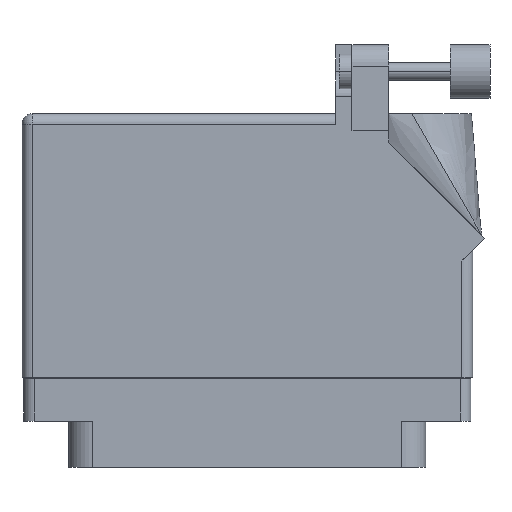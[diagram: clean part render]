
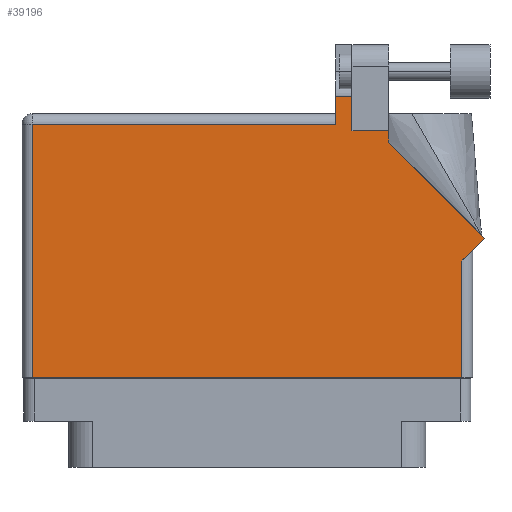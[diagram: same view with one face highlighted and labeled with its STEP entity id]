
A CAD part, front view. The second image highlights one B-rep face of the part: STEP entity #39196.
In plain terms, the highlighted face is planar.
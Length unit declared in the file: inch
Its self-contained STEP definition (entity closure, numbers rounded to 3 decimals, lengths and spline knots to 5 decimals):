
#301 = EDGE_CURVE ( 'NONE', #4619, #9848, #6210, .T. ) ;
#401 = DIRECTION ( 'NONE',  ( -1., 0., 0. ) ) ;
#438 = ORIENTED_EDGE ( 'NONE', *, *, #20001, .T. ) ;
#2689 = DIRECTION ( 'NONE',  ( 0., 1., 0. ) ) ;
#3340 = FACE_OUTER_BOUND ( 'NONE', #44465, .T. ) ;
#3405 = VECTOR ( 'NONE', #4112, 39.37008 ) ;
#3554 = EDGE_CURVE ( 'NONE', #15527, #26384, #39016, .T. ) ;
#4112 = DIRECTION ( 'NONE',  ( -1., 0., 0. ) ) ;
#4385 = ORIENTED_EDGE ( 'NONE', *, *, #27018, .T. ) ;
#4619 = VERTEX_POINT ( 'NONE', #20329 ) ;
#5492 = DIRECTION ( 'NONE',  ( 0.707, 0.707, 0. ) ) ;
#5613 = DIRECTION ( 'NONE',  ( -1., 0., 0. ) ) ;
#6042 = DIRECTION ( 'NONE',  ( -0.707, 0.707, 0. ) ) ;
#6210 = LINE ( 'NONE', #43360, #33582 ) ;
#6911 = EDGE_CURVE ( 'NONE', #28225, #24283, #7687, .T. ) ;
#7637 = VECTOR ( 'NONE', #14661, 39.37008 ) ;
#7687 = LINE ( 'NONE', #38793, #29189 ) ;
#8097 = LINE ( 'NONE', #26347, #3405 ) ;
#8151 = LINE ( 'NONE', #30465, #29691 ) ;
#9648 = ORIENTED_EDGE ( 'NONE', *, *, #18750, .T. ) ;
#9848 = VERTEX_POINT ( 'NONE', #14142 ) ;
#10163 = VECTOR ( 'NONE', #5492, 39.37008 ) ;
#10864 = ORIENTED_EDGE ( 'NONE', *, *, #29958, .T. ) ;
#11469 = LINE ( 'NONE', #13378, #44058 ) ;
#11847 = AXIS2_PLACEMENT_3D ( 'NONE', #15701, #12307, #5613 ) ;
#12105 = EDGE_CURVE ( 'NONE', #9848, #18011, #33276, .T. ) ;
#12145 = ORIENTED_EDGE ( 'NONE', *, *, #34560, .T. ) ;
#12307 = DIRECTION ( 'NONE',  ( 0., 0., -1. ) ) ;
#13378 = CARTESIAN_POINT ( 'NONE',  ( 1.37671, 0.70771, 0.455 ) ) ;
#13670 = CARTESIAN_POINT ( 'NONE',  ( 1.244, 0.575, 0.455 ) ) ;
#13788 = CARTESIAN_POINT ( 'NONE',  ( 0.82, 1.26442, 0.455 ) ) ;
#14142 = CARTESIAN_POINT ( 'NONE',  ( 0.607, 1.5315, 0.455 ) ) ;
#14661 = DIRECTION ( 'NONE',  ( -1., 0., 0. ) ) ;
#15088 = EDGE_CURVE ( 'NONE', #29782, #15527, #11469, .T. ) ;
#15526 = VECTOR ( 'NONE', #36649, 39.37008 ) ;
#15527 = VERTEX_POINT ( 'NONE', #13788 ) ;
#15701 = CARTESIAN_POINT ( 'NONE',  ( -1.306, 1.43, 0.455 ) ) ;
#16129 = VECTOR ( 'NONE', #34364, 39.37008 ) ;
#16530 = CARTESIAN_POINT ( 'NONE',  ( 1.306, 0.637, 0.455 ) ) ;
#18011 = VERTEX_POINT ( 'NONE', #37888 ) ;
#18750 = EDGE_CURVE ( 'NONE', #26384, #4619, #8151, .T. ) ;
#19612 = LINE ( 'NONE', #32923, #15526 ) ;
#20001 = EDGE_CURVE ( 'NONE', #28972, #47513, #19612, .T. ) ;
#20074 = CARTESIAN_POINT ( 'NONE',  ( 1.37671, 0.70771, 0.455 ) ) ;
#20146 = EDGE_CURVE ( 'NONE', #18011, #32366, #44082, .T. ) ;
#20329 = CARTESIAN_POINT ( 'NONE',  ( 0.607, 1.33, 0.455 ) ) ;
#20820 = CARTESIAN_POINT ( 'NONE',  ( 0.82, 1.26442, 0.455 ) ) ;
#21765 = VECTOR ( 'NONE', #27806, 39.37008 ) ;
#23316 = PLANE ( 'NONE',  #11847 ) ;
#24283 = VERTEX_POINT ( 'NONE', #31921 ) ;
#25215 = CARTESIAN_POINT ( 'NONE',  ( 1.244, -0.1, 0.455 ) ) ;
#26347 = CARTESIAN_POINT ( 'NONE',  ( -1.306, 1.368, 0.455 ) ) ;
#26384 = VERTEX_POINT ( 'NONE', #30199 ) ;
#26416 = LINE ( 'NONE', #16530, #10163 ) ;
#26766 = ORIENTED_EDGE ( 'NONE', *, *, #3554, .T. ) ;
#27018 = EDGE_CURVE ( 'NONE', #24283, #28972, #34591, .T. ) ;
#27426 = CARTESIAN_POINT ( 'NONE',  ( -1.244, 1.368, 0.455 ) ) ;
#27497 = DIRECTION ( 'NONE',  ( 0., 1., 0. ) ) ;
#27806 = DIRECTION ( 'NONE',  ( 1., 0., 0. ) ) ;
#28225 = VERTEX_POINT ( 'NONE', #27426 ) ;
#28299 = CARTESIAN_POINT ( 'NONE',  ( -1.306, -0.1, 0.455 ) ) ;
#28787 = ORIENTED_EDGE ( 'NONE', *, *, #301, .T. ) ;
#28972 = VERTEX_POINT ( 'NONE', #25215 ) ;
#29189 = VECTOR ( 'NONE', #31331, 39.37008 ) ;
#29691 = VECTOR ( 'NONE', #401, 39.37008 ) ;
#29782 = VERTEX_POINT ( 'NONE', #20074 ) ;
#29958 = EDGE_CURVE ( 'NONE', #32366, #28225, #8097, .T. ) ;
#30199 = CARTESIAN_POINT ( 'NONE',  ( 0.82, 1.33, 0.455 ) ) ;
#30465 = CARTESIAN_POINT ( 'NONE',  ( 0.82, 1.33, 0.455 ) ) ;
#31331 = DIRECTION ( 'NONE',  ( 0., -1., 0. ) ) ;
#31735 = CARTESIAN_POINT ( 'NONE',  ( 0.513, 1.368, 0.455 ) ) ;
#31921 = CARTESIAN_POINT ( 'NONE',  ( -1.244, -0.1, 0.455 ) ) ;
#32366 = VERTEX_POINT ( 'NONE', #31735 ) ;
#32923 = CARTESIAN_POINT ( 'NONE',  ( 1.244, 0.637, 0.455 ) ) ;
#33276 = LINE ( 'NONE', #40361, #7637 ) ;
#33582 = VECTOR ( 'NONE', #2689, 39.37008 ) ;
#34364 = DIRECTION ( 'NONE',  ( 0., -1., 0. ) ) ;
#34560 = EDGE_CURVE ( 'NONE', #47513, #29782, #26416, .T. ) ;
#34591 = LINE ( 'NONE', #28299, #21765 ) ;
#35527 = VECTOR ( 'NONE', #27497, 39.37008 ) ;
#35938 = ORIENTED_EDGE ( 'NONE', *, *, #15088, .T. ) ;
#36649 = DIRECTION ( 'NONE',  ( 0., 1., 0. ) ) ;
#37888 = CARTESIAN_POINT ( 'NONE',  ( 0.513, 1.5315, 0.455 ) ) ;
#38398 = CARTESIAN_POINT ( 'NONE',  ( 0.513, 1.43, 0.455 ) ) ;
#38793 = CARTESIAN_POINT ( 'NONE',  ( -1.244, -0.1, 0.455 ) ) ;
#39016 = LINE ( 'NONE', #20820, #35527 ) ;
#39196 = ADVANCED_FACE ( 'NONE', ( #3340 ), #23316, .F. ) ;
#40361 = CARTESIAN_POINT ( 'NONE',  ( 0.93777, 1.5315, 0.455 ) ) ;
#41078 = ORIENTED_EDGE ( 'NONE', *, *, #20146, .T. ) ;
#41750 = ORIENTED_EDGE ( 'NONE', *, *, #6911, .T. ) ;
#41781 = ORIENTED_EDGE ( 'NONE', *, *, #12105, .T. ) ;
#43360 = CARTESIAN_POINT ( 'NONE',  ( 0.607, 1.33, 0.455 ) ) ;
#44058 = VECTOR ( 'NONE', #6042, 39.37008 ) ;
#44082 = LINE ( 'NONE', #38398, #16129 ) ;
#44465 = EDGE_LOOP ( 'NONE', ( #28787, #41781, #41078, #10864, #41750, #4385, #438, #12145, #35938, #26766, #9648 ) ) ;
#47513 = VERTEX_POINT ( 'NONE', #13670 ) ;
